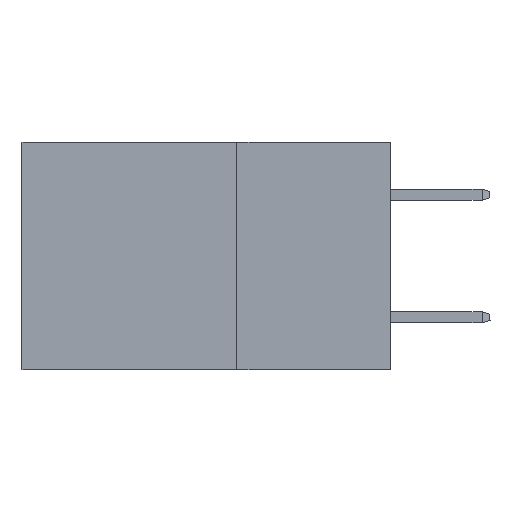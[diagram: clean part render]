
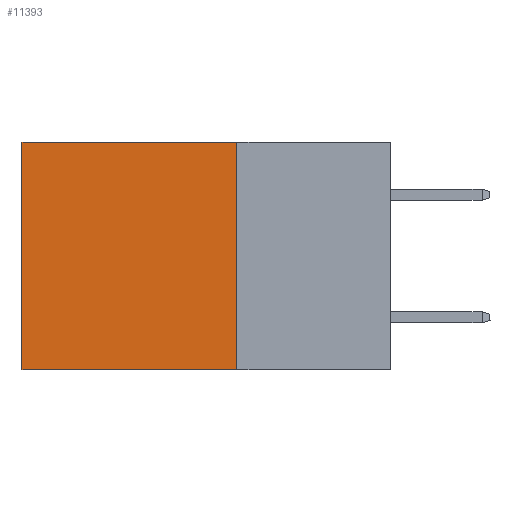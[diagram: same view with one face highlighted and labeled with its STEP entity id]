
A CAD part, left-side view. The second image highlights one B-rep face of the part: STEP entity #11393.
In plain terms, the highlighted planar face has unit normal (-1, 0, 0).
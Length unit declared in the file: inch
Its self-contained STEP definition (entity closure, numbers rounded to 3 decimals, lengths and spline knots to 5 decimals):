
#619 = DIRECTION ( 'NONE',  ( 0., 0., -1. ) ) ;
#1219 = EDGE_CURVE ( 'NONE', #17909, #10206, #7814, .T. ) ;
#1225 = EDGE_CURVE ( 'NONE', #13634, #2124, #10942, .T. ) ;
#1266 = LINE ( 'NONE', #1562, #12354 ) ;
#1562 = CARTESIAN_POINT ( 'NONE',  ( 0.2875, 0.25, -0.37 ) ) ;
#2124 = VERTEX_POINT ( 'NONE', #2561 ) ;
#2525 = DIRECTION ( 'NONE',  ( 0., 1., 0. ) ) ;
#2561 = CARTESIAN_POINT ( 'NONE',  ( 0.2875, 0.25, -0.37 ) ) ;
#3946 = CARTESIAN_POINT ( 'NONE',  ( 0.2875, 0.25, 0. ) ) ;
#5691 = FACE_OUTER_BOUND ( 'NONE', #6807, .T. ) ;
#6508 = CARTESIAN_POINT ( 'NONE',  ( 0.2875, 0.25, 0. ) ) ;
#6807 = EDGE_LOOP ( 'NONE', ( #10653, #11361, #14143, #12963 ) ) ;
#7814 = LINE ( 'NONE', #7919, #15556 ) ;
#7919 = CARTESIAN_POINT ( 'NONE',  ( 0.2875, 0.6, 0. ) ) ;
#9198 = VECTOR ( 'NONE', #2525, 39.37008 ) ;
#9387 = DIRECTION ( 'NONE',  ( 1., 0., 0. ) ) ;
#10206 = VERTEX_POINT ( 'NONE', #16436 ) ;
#10653 = ORIENTED_EDGE ( 'NONE', *, *, #1219, .T. ) ;
#10792 = DIRECTION ( 'NONE',  ( 0., 0., -1. ) ) ;
#10942 = LINE ( 'NONE', #6508, #14915 ) ;
#11361 = ORIENTED_EDGE ( 'NONE', *, *, #11855, .F. ) ;
#11393 = ADVANCED_FACE ( 'NONE', ( #5691 ), #15004, .F. ) ;
#11855 = EDGE_CURVE ( 'NONE', #2124, #10206, #1266, .T. ) ;
#12181 = CARTESIAN_POINT ( 'NONE',  ( 0.2875, 0.25, 0. ) ) ;
#12354 = VECTOR ( 'NONE', #13128, 39.37008 ) ;
#12963 = ORIENTED_EDGE ( 'NONE', *, *, #14599, .T. ) ;
#13128 = DIRECTION ( 'NONE',  ( 0., 1., 0. ) ) ;
#13149 = AXIS2_PLACEMENT_3D ( 'NONE', #12181, #9387, #619 ) ;
#13448 = LINE ( 'NONE', #3946, #9198 ) ;
#13634 = VERTEX_POINT ( 'NONE', #17542 ) ;
#14143 = ORIENTED_EDGE ( 'NONE', *, *, #1225, .F. ) ;
#14457 = CARTESIAN_POINT ( 'NONE',  ( 0.2875, 0.6, 0. ) ) ;
#14599 = EDGE_CURVE ( 'NONE', #13634, #17909, #13448, .T. ) ;
#14915 = VECTOR ( 'NONE', #10792, 39.37008 ) ;
#15004 = PLANE ( 'NONE',  #13149 ) ;
#15556 = VECTOR ( 'NONE', #17797, 39.37008 ) ;
#16436 = CARTESIAN_POINT ( 'NONE',  ( 0.2875, 0.6, -0.37 ) ) ;
#17542 = CARTESIAN_POINT ( 'NONE',  ( 0.2875, 0.25, 0. ) ) ;
#17797 = DIRECTION ( 'NONE',  ( 0., 0., -1. ) ) ;
#17909 = VERTEX_POINT ( 'NONE', #14457 ) ;
